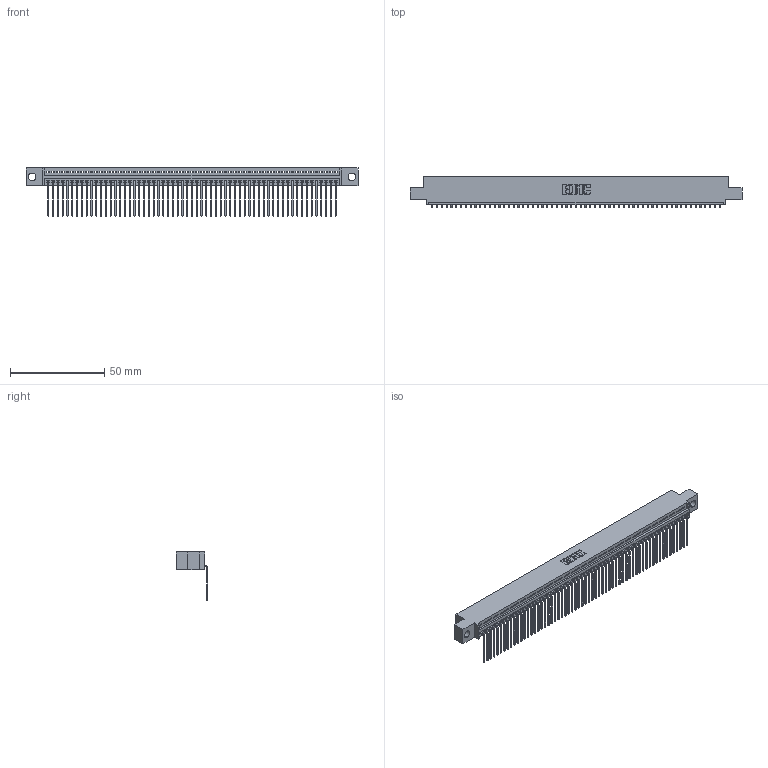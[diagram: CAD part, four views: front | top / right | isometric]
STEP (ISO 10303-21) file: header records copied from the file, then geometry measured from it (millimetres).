
FILE_DESCRIPTION (( 'STEP AP203' ), '1' );
FILE_NAME ('395-061-559-404.STEP', '2021-05-31T21:52:32', ( '' ), ( '' ), 'SwSTEP 2.0', 'SolidWorks 2020', '' );
FILE_SCHEMA (( 'CONFIG_CONTROL_DESIGN' ));
Length unit declared in the file: inch
Products named in the file (3): 345 Part_0.110 Offset - 0.156 Dia-TI; 395-061-559-404; 345-292-001_558 559 Tail - 1
Assembly tree (62 placements, depth 2):
  395-061-559-404
    345 Part_0.110 Offset - 0.156 Dia-TI
    345-292-001_558 559 Tail - 1  x61
Bounding box: 176.15 x 16.75 x 25.53 mm (x, y, z)
Volume: 16910.4 mm3; surface area: 23849.2 mm2
Topology: 62 solids, 62 shells, 3804 faces, 11491 edges, 7578 vertices
Faces by surface type: plane 2660, cylinder 1144
Entity records: 43987 total; most frequent: CARTESIAN_POINT 7629, ORIENTED_EDGE 7622, DIRECTION 6633, EDGE_CURVE 3811, VECTOR 3435, LINE 3435, VERTEX_POINT 2538, AXIS2_PLACEMENT_3D 1599
